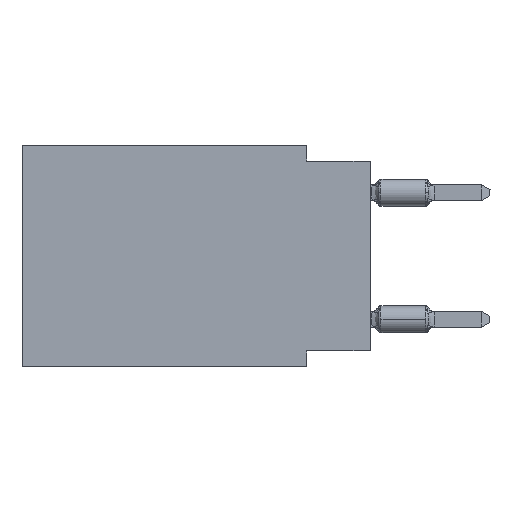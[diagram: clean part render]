
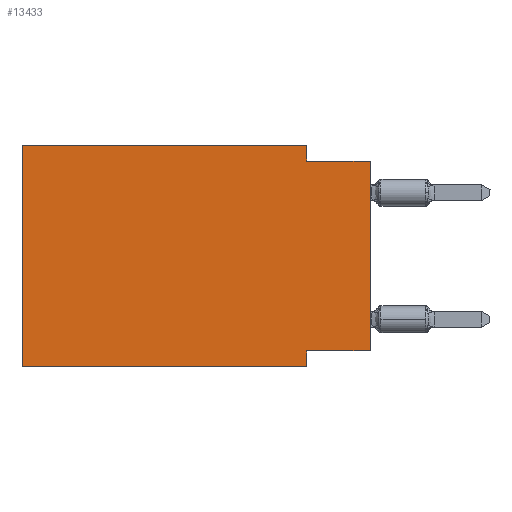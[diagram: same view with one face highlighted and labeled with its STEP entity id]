
A CAD part, left-side view. The second image highlights one B-rep face of the part: STEP entity #13433.
In plain terms, the highlighted planar face has unit normal (-1, 0, 0).
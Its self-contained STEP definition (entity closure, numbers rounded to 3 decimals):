
#184 = LINE ( 'NONE', #7160, #5267 ) ;
#482 = CARTESIAN_POINT ( 'NONE',  ( 0., 0., -8.255 ) ) ;
#767 = VERTEX_POINT ( 'NONE', #8606 ) ;
#791 = LINE ( 'NONE', #9565, #14847 ) ;
#824 = CARTESIAN_POINT ( 'NONE',  ( 0., 2.54, -8.89 ) ) ;
#1032 = DIRECTION ( 'NONE',  ( 0., 0., -1. ) ) ;
#1033 = VERTEX_POINT ( 'NONE', #10872 ) ;
#1103 = LINE ( 'NONE', #16781, #1277 ) ;
#1175 = VERTEX_POINT ( 'NONE', #2920 ) ;
#1277 = VECTOR ( 'NONE', #3852, 1000. ) ;
#1309 = VERTEX_POINT ( 'NONE', #824 ) ;
#1571 = ORIENTED_EDGE ( 'NONE', *, *, #13960, .F. ) ;
#1834 = EDGE_CURVE ( 'NONE', #1175, #11944, #2587, .T. ) ;
#2587 = LINE ( 'NONE', #15244, #12921 ) ;
#2619 = VECTOR ( 'NONE', #4838, 1000. ) ;
#2795 = VERTEX_POINT ( 'NONE', #5553 ) ;
#2920 = CARTESIAN_POINT ( 'NONE',  ( 0., 13.97, 0. ) ) ;
#3055 = ORIENTED_EDGE ( 'NONE', *, *, #15101, .F. ) ;
#3109 = ORIENTED_EDGE ( 'NONE', *, *, #11675, .F. ) ;
#3442 = EDGE_CURVE ( 'NONE', #767, #8403, #5417, .T. ) ;
#3852 = DIRECTION ( 'NONE',  ( 0., 0., -1. ) ) ;
#4786 = VECTOR ( 'NONE', #7134, 1000. ) ;
#4838 = DIRECTION ( 'NONE',  ( 0., -1., 0. ) ) ;
#5043 = DIRECTION ( 'NONE',  ( 0., 0., 1. ) ) ;
#5267 = VECTOR ( 'NONE', #15755, 1000. ) ;
#5311 = CARTESIAN_POINT ( 'NONE',  ( 0., 2.54, 0. ) ) ;
#5331 = DIRECTION ( 'NONE',  ( 0., -1., 0. ) ) ;
#5417 = LINE ( 'NONE', #13723, #6732 ) ;
#5553 = CARTESIAN_POINT ( 'NONE',  ( 0., 13.97, -8.89 ) ) ;
#6232 = DIRECTION ( 'NONE',  ( 0., 1., 0. ) ) ;
#6579 = VECTOR ( 'NONE', #6232, 1000. ) ;
#6703 = ORIENTED_EDGE ( 'NONE', *, *, #1834, .F. ) ;
#6732 = VECTOR ( 'NONE', #5043, 1000. ) ;
#7134 = DIRECTION ( 'NONE',  ( 0., 0., 1. ) ) ;
#7160 = CARTESIAN_POINT ( 'NONE',  ( 0., 2.54, -8.89 ) ) ;
#8403 = VERTEX_POINT ( 'NONE', #15560 ) ;
#8606 = CARTESIAN_POINT ( 'NONE',  ( 0., 0., -8.255 ) ) ;
#8816 = CARTESIAN_POINT ( 'NONE',  ( 0., 13.97, 0. ) ) ;
#8922 = LINE ( 'NONE', #8816, #4786 ) ;
#9565 = CARTESIAN_POINT ( 'NONE',  ( 0., 13.97, -8.89 ) ) ;
#9991 = CARTESIAN_POINT ( 'NONE',  ( 0., 13.97, 0. ) ) ;
#10680 = ORIENTED_EDGE ( 'NONE', *, *, #3442, .T. ) ;
#10872 = CARTESIAN_POINT ( 'NONE',  ( 0., 2.54, -8.255 ) ) ;
#11675 = EDGE_CURVE ( 'NONE', #18331, #8403, #13524, .T. ) ;
#11801 = LINE ( 'NONE', #482, #6579 ) ;
#11944 = VERTEX_POINT ( 'NONE', #5311 ) ;
#12011 = AXIS2_PLACEMENT_3D ( 'NONE', #9991, #18304, #1032 ) ;
#12075 = ORIENTED_EDGE ( 'NONE', *, *, #17273, .F. ) ;
#12392 = DIRECTION ( 'NONE',  ( 0., -1., 0. ) ) ;
#12921 = VECTOR ( 'NONE', #5331, 1000. ) ;
#13222 = EDGE_CURVE ( 'NONE', #767, #1033, #11801, .T. ) ;
#13433 = ADVANCED_FACE ( 'NONE', ( #14061 ), #17166, .F. ) ;
#13524 = LINE ( 'NONE', #17761, #2619 ) ;
#13723 = CARTESIAN_POINT ( 'NONE',  ( 0., 0., 0. ) ) ;
#13960 = EDGE_CURVE ( 'NONE', #2795, #1175, #8922, .T. ) ;
#14022 = ORIENTED_EDGE ( 'NONE', *, *, #13222, .F. ) ;
#14061 = FACE_OUTER_BOUND ( 'NONE', #15236, .T. ) ;
#14389 = ORIENTED_EDGE ( 'NONE', *, *, #14678, .T. ) ;
#14678 = EDGE_CURVE ( 'NONE', #2795, #1309, #791, .T. ) ;
#14847 = VECTOR ( 'NONE', #12392, 1000. ) ;
#15101 = EDGE_CURVE ( 'NONE', #11944, #18331, #1103, .T. ) ;
#15236 = EDGE_LOOP ( 'NONE', ( #10680, #3109, #3055, #6703, #1571, #14389, #12075, #14022 ) ) ;
#15244 = CARTESIAN_POINT ( 'NONE',  ( 0., 13.97, 0. ) ) ;
#15560 = CARTESIAN_POINT ( 'NONE',  ( 0., 0., -0.635 ) ) ;
#15755 = DIRECTION ( 'NONE',  ( 0., 0., -1. ) ) ;
#16781 = CARTESIAN_POINT ( 'NONE',  ( 0., 2.54, 0. ) ) ;
#17166 = PLANE ( 'NONE',  #12011 ) ;
#17273 = EDGE_CURVE ( 'NONE', #1033, #1309, #184, .T. ) ;
#17761 = CARTESIAN_POINT ( 'NONE',  ( 0., 0., -0.635 ) ) ;
#18054 = CARTESIAN_POINT ( 'NONE',  ( 0., 2.54, -0.635 ) ) ;
#18304 = DIRECTION ( 'NONE',  ( 1., 0., 0. ) ) ;
#18331 = VERTEX_POINT ( 'NONE', #18054 ) ;
